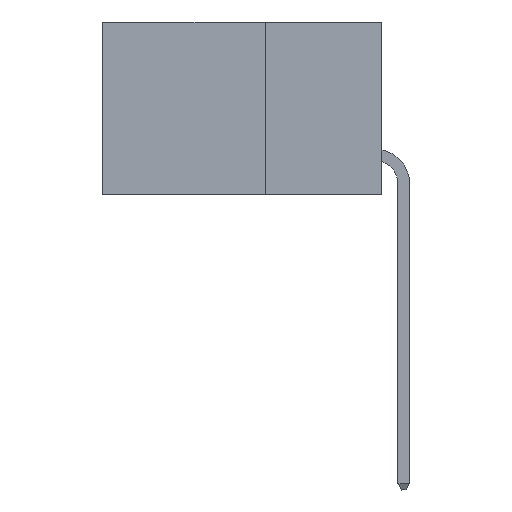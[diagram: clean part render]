
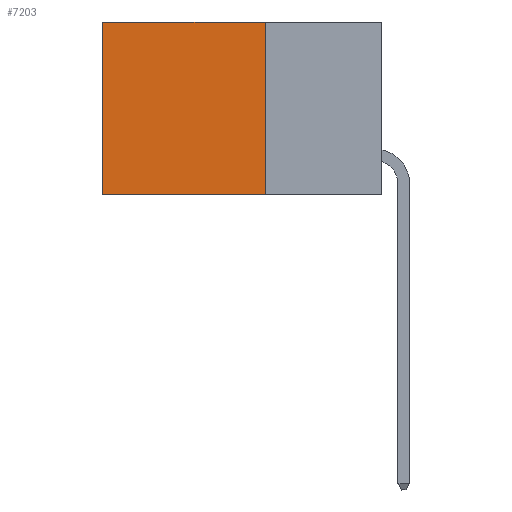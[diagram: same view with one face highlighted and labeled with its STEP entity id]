
A CAD part, left-side view. The second image highlights one B-rep face of the part: STEP entity #7203.
In plain terms, the highlighted planar face has unit normal (-1, 0, 0).
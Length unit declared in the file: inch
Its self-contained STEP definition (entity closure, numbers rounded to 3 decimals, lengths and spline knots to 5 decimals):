
#3123 = EDGE_CURVE ( 'NONE', #14662, #30757, #17491, .T. ) ;
#6658 = VERTEX_POINT ( 'NONE', #32493 ) ;
#7203 = ADVANCED_FACE ( 'NONE', ( #26825 ), #36910, .F. ) ;
#7245 = EDGE_CURVE ( 'NONE', #6658, #30757, #8740, .T. ) ;
#8624 = EDGE_LOOP ( 'NONE', ( #38963, #17640, #28102, #33653 ) ) ;
#8740 = LINE ( 'NONE', #25534, #20673 ) ;
#9577 = CARTESIAN_POINT ( 'NONE',  ( 0.2875, 0.25, 0. ) ) ;
#10338 = VECTOR ( 'NONE', #37362, 39.37008 ) ;
#11880 = DIRECTION ( 'NONE',  ( 0., 0., -1. ) ) ;
#14586 = CARTESIAN_POINT ( 'NONE',  ( 0.2875, 0.6, -0.37 ) ) ;
#14662 = VERTEX_POINT ( 'NONE', #18719 ) ;
#17491 = LINE ( 'NONE', #21990, #19830 ) ;
#17640 = ORIENTED_EDGE ( 'NONE', *, *, #7245, .F. ) ;
#18189 = CARTESIAN_POINT ( 'NONE',  ( 0.2875, 0.25, 0. ) ) ;
#18627 = EDGE_CURVE ( 'NONE', #38940, #14662, #20362, .T. ) ;
#18719 = CARTESIAN_POINT ( 'NONE',  ( 0.2875, 0.6, 0. ) ) ;
#19389 = DIRECTION ( 'NONE',  ( 0., 0., -1. ) ) ;
#19830 = VECTOR ( 'NONE', #19389, 39.37008 ) ;
#19894 = AXIS2_PLACEMENT_3D ( 'NONE', #9577, #40785, #36532 ) ;
#20362 = LINE ( 'NONE', #41368, #10338 ) ;
#20673 = VECTOR ( 'NONE', #44408, 39.37008 ) ;
#21990 = CARTESIAN_POINT ( 'NONE',  ( 0.2875, 0.6, 0. ) ) ;
#25534 = CARTESIAN_POINT ( 'NONE',  ( 0.2875, 0.25, -0.37 ) ) ;
#26299 = EDGE_CURVE ( 'NONE', #38940, #6658, #27366, .T. ) ;
#26825 = FACE_OUTER_BOUND ( 'NONE', #8624, .T. ) ;
#27366 = LINE ( 'NONE', #41054, #36317 ) ;
#28102 = ORIENTED_EDGE ( 'NONE', *, *, #26299, .F. ) ;
#30757 = VERTEX_POINT ( 'NONE', #14586 ) ;
#32493 = CARTESIAN_POINT ( 'NONE',  ( 0.2875, 0.25, -0.37 ) ) ;
#33653 = ORIENTED_EDGE ( 'NONE', *, *, #18627, .T. ) ;
#36317 = VECTOR ( 'NONE', #11880, 39.37008 ) ;
#36532 = DIRECTION ( 'NONE',  ( 0., 0., -1. ) ) ;
#36910 = PLANE ( 'NONE',  #19894 ) ;
#37362 = DIRECTION ( 'NONE',  ( 0., 1., 0. ) ) ;
#38940 = VERTEX_POINT ( 'NONE', #18189 ) ;
#38963 = ORIENTED_EDGE ( 'NONE', *, *, #3123, .T. ) ;
#40785 = DIRECTION ( 'NONE',  ( 1., 0., 0. ) ) ;
#41054 = CARTESIAN_POINT ( 'NONE',  ( 0.2875, 0.25, 0. ) ) ;
#41368 = CARTESIAN_POINT ( 'NONE',  ( 0.2875, 0.25, 0. ) ) ;
#44408 = DIRECTION ( 'NONE',  ( 0., 1., 0. ) ) ;
